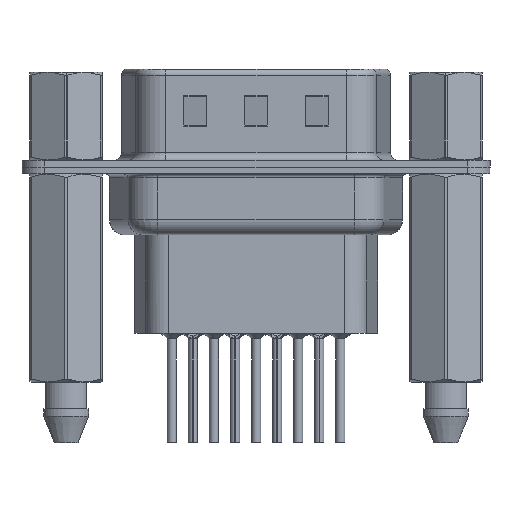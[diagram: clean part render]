
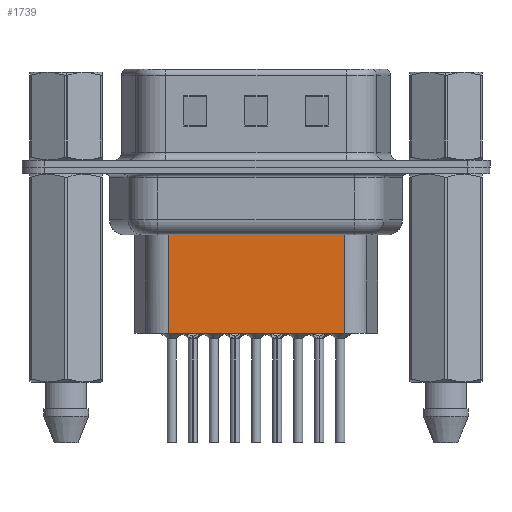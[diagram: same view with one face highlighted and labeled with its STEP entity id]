
A CAD part, front view. The second image highlights one B-rep face of the part: STEP entity #1739.
In plain terms, the highlighted planar face has unit normal (0, -1, 0).
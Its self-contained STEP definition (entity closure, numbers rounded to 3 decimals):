
#517 = CARTESIAN_POINT ( 'NONE',  ( 6.706, -3.5, -10.95 ) ) ;
#556 = ORIENTED_EDGE ( 'NONE', *, *, #14801, .F. ) ;
#1739 = ADVANCED_FACE ( 'NONE', ( #26018 ), #24161, .T. ) ;
#2001 = LINE ( 'NONE', #17996, #15014 ) ;
#2883 = LINE ( 'NONE', #517, #22468 ) ;
#4632 = VERTEX_POINT ( 'NONE', #25679 ) ;
#5712 = DIRECTION ( 'NONE',  ( 0., 0., -1. ) ) ;
#5816 = VERTEX_POINT ( 'NONE', #11895 ) ;
#6536 = ORIENTED_EDGE ( 'NONE', *, *, #10904, .T. ) ;
#7685 = DIRECTION ( 'NONE',  ( 1., 0., 0. ) ) ;
#8677 = ORIENTED_EDGE ( 'NONE', *, *, #15444, .T. ) ;
#9431 = CARTESIAN_POINT ( 'NONE',  ( 6.706, -3.5, -4.097 ) ) ;
#9563 = LINE ( 'NONE', #25389, #20085 ) ;
#10731 = ORIENTED_EDGE ( 'NONE', *, *, #24694, .F. ) ;
#10904 = EDGE_CURVE ( 'NONE', #14768, #5816, #2001, .T. ) ;
#11274 = DIRECTION ( 'NONE',  ( -1., 0., 0. ) ) ;
#11895 = CARTESIAN_POINT ( 'NONE',  ( 6.706, -3.5, -10.95 ) ) ;
#13809 = DIRECTION ( 'NONE',  ( 0., 0., -1. ) ) ;
#14039 = CARTESIAN_POINT ( 'NONE',  ( 6.706, -3.5, -3.1 ) ) ;
#14768 = VERTEX_POINT ( 'NONE', #9431 ) ;
#14801 = EDGE_CURVE ( 'NONE', #15939, #4632, #9563, .T. ) ;
#15014 = VECTOR ( 'NONE', #13809, 1000. ) ;
#15444 = EDGE_CURVE ( 'NONE', #15939, #14768, #24974, .T. ) ;
#15546 = VECTOR ( 'NONE', #11274, 1000. ) ;
#15939 = VERTEX_POINT ( 'NONE', #24939 ) ;
#17996 = CARTESIAN_POINT ( 'NONE',  ( 6.706, -3.5, -3.1 ) ) ;
#19302 = CARTESIAN_POINT ( 'NONE',  ( 6.459, -3.5, -4.097 ) ) ;
#20085 = VECTOR ( 'NONE', #5712, 1000. ) ;
#21123 = AXIS2_PLACEMENT_3D ( 'NONE', #14039, #25756, #7685 ) ;
#22468 = VECTOR ( 'NONE', #22686, 1000. ) ;
#22686 = DIRECTION ( 'NONE',  ( -1., 0., 0. ) ) ;
#23013 = EDGE_LOOP ( 'NONE', ( #556, #8677, #6536, #10731 ) ) ;
#24161 = PLANE ( 'NONE',  #21123 ) ;
#24694 = EDGE_CURVE ( 'NONE', #4632, #5816, #2883, .T. ) ;
#24939 = CARTESIAN_POINT ( 'NONE',  ( 18.294, -3.5, -4.097 ) ) ;
#24974 = LINE ( 'NONE', #19302, #15546 ) ;
#25389 = CARTESIAN_POINT ( 'NONE',  ( 18.294, -3.5, -3.1 ) ) ;
#25679 = CARTESIAN_POINT ( 'NONE',  ( 18.294, -3.5, -10.95 ) ) ;
#25756 = DIRECTION ( 'NONE',  ( 0., -1., 0. ) ) ;
#26018 = FACE_OUTER_BOUND ( 'NONE', #23013, .T. ) ;
